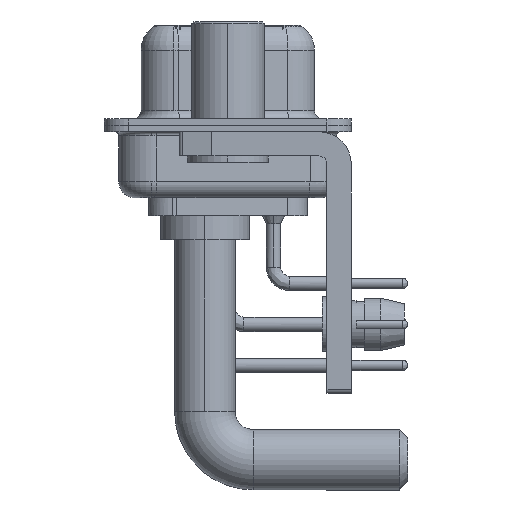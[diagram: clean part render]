
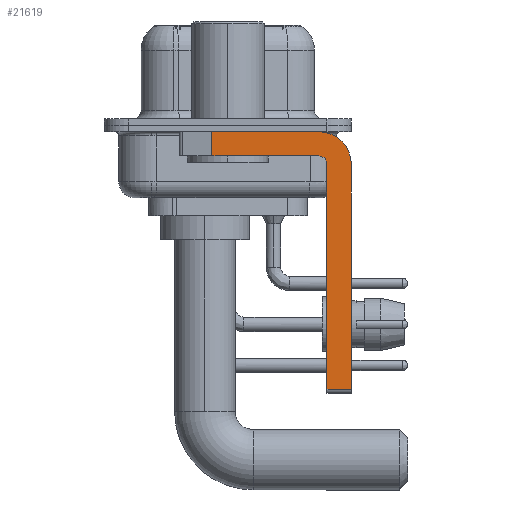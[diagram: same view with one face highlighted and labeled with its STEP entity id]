
A CAD part, left-side view. The second image highlights one B-rep face of the part: STEP entity #21619.
In plain terms, the highlighted planar face has unit normal (-1, 0, 0).
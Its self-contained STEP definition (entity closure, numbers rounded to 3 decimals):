
#244 = AXIS2_PLACEMENT_3D ( 'NONE', #33151, #25117, #33327 ) ;
#509 = DIRECTION ( 'NONE',  ( 1., 0., 0. ) ) ;
#902 = EDGE_CURVE ( 'NONE', #6063, #27635, #10393, .T. ) ;
#2139 = CARTESIAN_POINT ( 'NONE',  ( -2.9, -5.65, -16.35 ) ) ;
#2542 = LINE ( 'NONE', #27916, #30588 ) ;
#2882 = LINE ( 'NONE', #22051, #9940 ) ;
#2917 = DIRECTION ( 'NONE',  ( 0., 1., 0. ) ) ;
#3044 = DIRECTION ( 'NONE',  ( 0., 0., -1. ) ) ;
#3297 = CARTESIAN_POINT ( 'NONE',  ( -2.9, -7.65, -2.4 ) ) ;
#3749 = VECTOR ( 'NONE', #10995, 1000. ) ;
#4050 = ORIENTED_EDGE ( 'NONE', *, *, #31671, .T. ) ;
#5371 = ORIENTED_EDGE ( 'NONE', *, *, #31387, .F. ) ;
#6063 = VERTEX_POINT ( 'NONE', #22188 ) ;
#7293 = VECTOR ( 'NONE', #18231, 1000. ) ;
#7311 = VECTOR ( 'NONE', #27817, 1000. ) ;
#7587 = EDGE_CURVE ( 'NONE', #20883, #14565, #2882, .T. ) ;
#8053 = AXIS2_PLACEMENT_3D ( 'NONE', #29804, #15955, #32002 ) ;
#8324 = CARTESIAN_POINT ( 'NONE',  ( -2.9, -5.65, -0.4 ) ) ;
#8706 = CARTESIAN_POINT ( 'NONE',  ( -2.9, -7.65, -2.4 ) ) ;
#8885 = LINE ( 'NONE', #8706, #13232 ) ;
#9062 = EDGE_CURVE ( 'NONE', #27744, #28226, #13173, .T. ) ;
#9724 = DIRECTION ( 'NONE',  ( 0., 0., -1. ) ) ;
#9767 = CARTESIAN_POINT ( 'NONE',  ( -2.9, -7.65, -16.35 ) ) ;
#9826 = EDGE_CURVE ( 'NONE', #28226, #18594, #8885, .T. ) ;
#9940 = VECTOR ( 'NONE', #11283, 1000. ) ;
#10233 = EDGE_CURVE ( 'NONE', #20883, #27744, #16904, .T. ) ;
#10393 = CIRCLE ( 'NONE', #8053, 0.5 ) ;
#10995 = DIRECTION ( 'NONE',  ( 0., 0., 1. ) ) ;
#11283 = DIRECTION ( 'NONE',  ( 0., 0., -1. ) ) ;
#11539 = LINE ( 'NONE', #22659, #3749 ) ;
#12175 = ORIENTED_EDGE ( 'NONE', *, *, #9062, .F. ) ;
#12532 = ORIENTED_EDGE ( 'NONE', *, *, #9826, .F. ) ;
#13173 = CIRCLE ( 'NONE', #22494, 2. ) ;
#13232 = VECTOR ( 'NONE', #3044, 1000. ) ;
#13472 = ORIENTED_EDGE ( 'NONE', *, *, #10233, .F. ) ;
#14565 = VERTEX_POINT ( 'NONE', #34693 ) ;
#15661 = ORIENTED_EDGE ( 'NONE', *, *, #7587, .T. ) ;
#15713 = VERTEX_POINT ( 'NONE', #33988 ) ;
#15955 = DIRECTION ( 'NONE',  ( -1., 0., 0. ) ) ;
#16904 = LINE ( 'NONE', #33843, #7311 ) ;
#18231 = DIRECTION ( 'NONE',  ( 0., -1., 0. ) ) ;
#18594 = VERTEX_POINT ( 'NONE', #9767 ) ;
#19047 = ORIENTED_EDGE ( 'NONE', *, *, #902, .F. ) ;
#20883 = VERTEX_POINT ( 'NONE', #31223 ) ;
#21619 = ADVANCED_FACE ( 'NONE', ( #24745 ), #25466, .F. ) ;
#22051 = CARTESIAN_POINT ( 'NONE',  ( -2.9, 0.978, -1.9 ) ) ;
#22188 = CARTESIAN_POINT ( 'NONE',  ( -2.9, -6.15, -2.4 ) ) ;
#22494 = AXIS2_PLACEMENT_3D ( 'NONE', #25496, #509, #9724 ) ;
#22659 = CARTESIAN_POINT ( 'NONE',  ( -2.9, -6.15, -16.6 ) ) ;
#24745 = FACE_OUTER_BOUND ( 'NONE', #27342, .T. ) ;
#25117 = DIRECTION ( 'NONE',  ( 1., 0., 0. ) ) ;
#25466 = PLANE ( 'NONE',  #244 ) ;
#25496 = CARTESIAN_POINT ( 'NONE',  ( -2.9, -5.65, -2.4 ) ) ;
#27137 = LINE ( 'NONE', #2139, #7293 ) ;
#27342 = EDGE_LOOP ( 'NONE', ( #13472, #15661, #5371, #19047, #33081, #4050, #12532, #12175 ) ) ;
#27635 = VERTEX_POINT ( 'NONE', #29849 ) ;
#27744 = VERTEX_POINT ( 'NONE', #8324 ) ;
#27817 = DIRECTION ( 'NONE',  ( 0., -1., 0. ) ) ;
#27916 = CARTESIAN_POINT ( 'NONE',  ( -2.9, -5.65, -1.9 ) ) ;
#28226 = VERTEX_POINT ( 'NONE', #3297 ) ;
#29804 = CARTESIAN_POINT ( 'NONE',  ( -2.9, -5.65, -2.4 ) ) ;
#29849 = CARTESIAN_POINT ( 'NONE',  ( -2.9, -5.65, -1.9 ) ) ;
#30588 = VECTOR ( 'NONE', #2917, 1000. ) ;
#30891 = EDGE_CURVE ( 'NONE', #15713, #6063, #11539, .T. ) ;
#31223 = CARTESIAN_POINT ( 'NONE',  ( -2.9, 0.978, -0.4 ) ) ;
#31387 = EDGE_CURVE ( 'NONE', #27635, #14565, #2542, .T. ) ;
#31671 = EDGE_CURVE ( 'NONE', #15713, #18594, #27137, .T. ) ;
#32002 = DIRECTION ( 'NONE',  ( 0., 0., 1. ) ) ;
#33081 = ORIENTED_EDGE ( 'NONE', *, *, #30891, .F. ) ;
#33151 = CARTESIAN_POINT ( 'NONE',  ( -2.9, -5.65, -2.4 ) ) ;
#33327 = DIRECTION ( 'NONE',  ( 0., 0., -1. ) ) ;
#33843 = CARTESIAN_POINT ( 'NONE',  ( -2.9, 3., -0.4 ) ) ;
#33988 = CARTESIAN_POINT ( 'NONE',  ( -2.9, -6.15, -16.35 ) ) ;
#34693 = CARTESIAN_POINT ( 'NONE',  ( -2.9, 0.978, -1.9 ) ) ;
